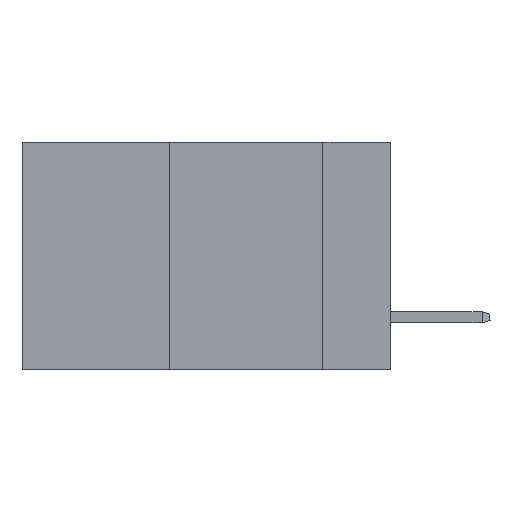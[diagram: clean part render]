
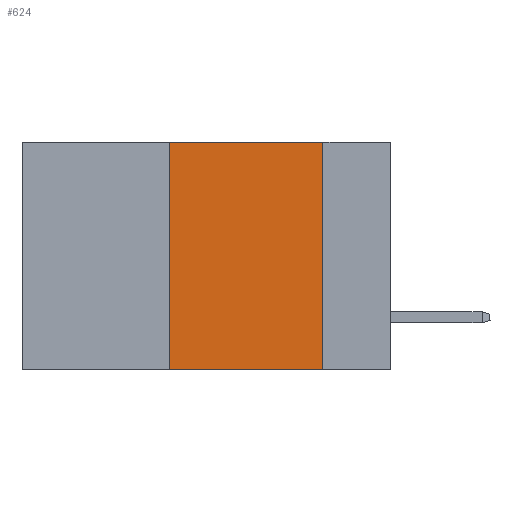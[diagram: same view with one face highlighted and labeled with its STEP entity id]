
A CAD part, left-side view. The second image highlights one B-rep face of the part: STEP entity #624.
In plain terms, the highlighted planar face has unit normal (-1, 0, 0).
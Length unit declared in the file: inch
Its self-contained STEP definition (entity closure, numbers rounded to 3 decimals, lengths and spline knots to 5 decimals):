
#205 = DIRECTION ( 'NONE',  ( 0., -1., 0. ) ) ;
#624 = ADVANCED_FACE ( 'NONE', ( #19568 ), #11613, .F. ) ;
#1005 = CARTESIAN_POINT ( 'NONE',  ( 0., 0.11, 0. ) ) ;
#1145 = CARTESIAN_POINT ( 'NONE',  ( 0., 0.36, 0. ) ) ;
#1344 = DIRECTION ( 'NONE',  ( 0., 0., -1. ) ) ;
#1363 = DIRECTION ( 'NONE',  ( 0., 0., 1. ) ) ;
#2809 = VERTEX_POINT ( 'NONE', #7190 ) ;
#5895 = VERTEX_POINT ( 'NONE', #17847 ) ;
#6024 = VECTOR ( 'NONE', #11348, 39.37008 ) ;
#6045 = VERTEX_POINT ( 'NONE', #1005 ) ;
#6129 = DIRECTION ( 'NONE',  ( 1., 0., 0. ) ) ;
#6212 = DIRECTION ( 'NONE',  ( 0., 0., -1. ) ) ;
#7190 = CARTESIAN_POINT ( 'NONE',  ( 0., 0.11, -0.37 ) ) ;
#7596 = LINE ( 'NONE', #1145, #21227 ) ;
#7978 = CARTESIAN_POINT ( 'NONE',  ( 0., 0.6, -0.37 ) ) ;
#8194 = EDGE_CURVE ( 'NONE', #15351, #2809, #17411, .T. ) ;
#8835 = EDGE_CURVE ( 'NONE', #5895, #6045, #15735, .T. ) ;
#9880 = CARTESIAN_POINT ( 'NONE',  ( 0., 0.6, 0. ) ) ;
#10877 = EDGE_CURVE ( 'NONE', #15351, #5895, #7596, .T. ) ;
#10895 = CARTESIAN_POINT ( 'NONE',  ( 0., 0.6, 0. ) ) ;
#11070 = CARTESIAN_POINT ( 'NONE',  ( 0., 0.36, -0.37 ) ) ;
#11348 = DIRECTION ( 'NONE',  ( 0., -1., 0. ) ) ;
#11480 = EDGE_LOOP ( 'NONE', ( #13314, #19556, #21739, #15874 ) ) ;
#11613 = PLANE ( 'NONE',  #14296 ) ;
#12050 = CARTESIAN_POINT ( 'NONE',  ( 0., 0.11, 0. ) ) ;
#13291 = EDGE_CURVE ( 'NONE', #6045, #2809, #14989, .T. ) ;
#13307 = VECTOR ( 'NONE', #1344, 39.37008 ) ;
#13314 = ORIENTED_EDGE ( 'NONE', *, *, #13291, .F. ) ;
#14296 = AXIS2_PLACEMENT_3D ( 'NONE', #9880, #6129, #6212 ) ;
#14989 = LINE ( 'NONE', #12050, #13307 ) ;
#15351 = VERTEX_POINT ( 'NONE', #11070 ) ;
#15735 = LINE ( 'NONE', #10895, #17392 ) ;
#15874 = ORIENTED_EDGE ( 'NONE', *, *, #8194, .T. ) ;
#17392 = VECTOR ( 'NONE', #205, 39.37008 ) ;
#17411 = LINE ( 'NONE', #7978, #6024 ) ;
#17847 = CARTESIAN_POINT ( 'NONE',  ( 0., 0.36, 0. ) ) ;
#19556 = ORIENTED_EDGE ( 'NONE', *, *, #8835, .F. ) ;
#19568 = FACE_OUTER_BOUND ( 'NONE', #11480, .T. ) ;
#21227 = VECTOR ( 'NONE', #1363, 39.37008 ) ;
#21739 = ORIENTED_EDGE ( 'NONE', *, *, #10877, .F. ) ;
